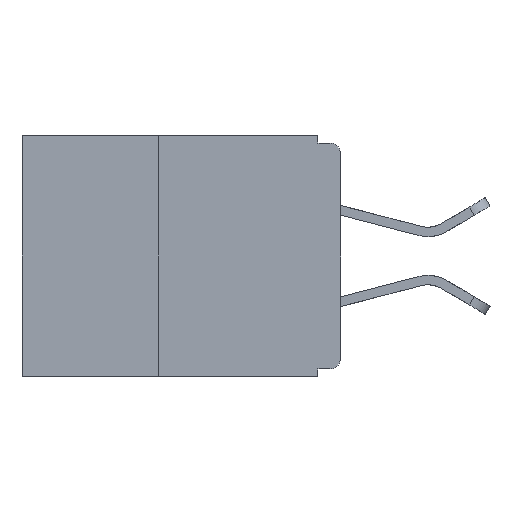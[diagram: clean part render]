
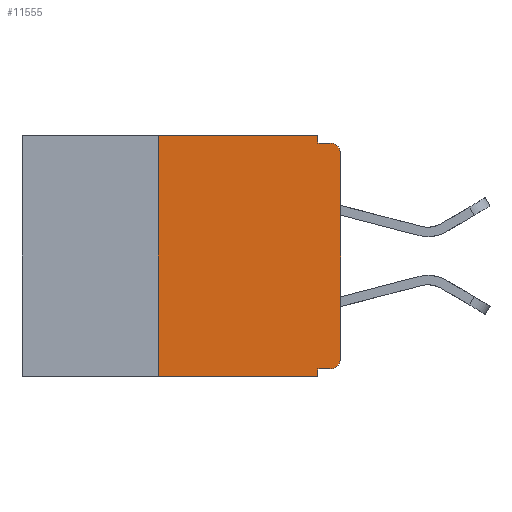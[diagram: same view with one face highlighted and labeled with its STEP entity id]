
A CAD part, left-side view. The second image highlights one B-rep face of the part: STEP entity #11555.
In plain terms, the highlighted planar face has unit normal (-1, 0, 0).
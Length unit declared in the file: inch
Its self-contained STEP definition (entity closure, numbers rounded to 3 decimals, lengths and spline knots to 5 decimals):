
#60 = LINE ( 'NONE', #8432, #3151 ) ;
#147 = ORIENTED_EDGE ( 'NONE', *, *, #15149, .F. ) ;
#393 = ORIENTED_EDGE ( 'NONE', *, *, #1273, .F. ) ;
#657 = VERTEX_POINT ( 'NONE', #5292 ) ;
#815 = LINE ( 'NONE', #12244, #10987 ) ;
#830 = LINE ( 'NONE', #1313, #14012 ) ;
#831 = EDGE_CURVE ( 'NONE', #12390, #9923, #12982, .T. ) ;
#835 = ORIENTED_EDGE ( 'NONE', *, *, #831, .F. ) ;
#950 = VERTEX_POINT ( 'NONE', #1779 ) ;
#1273 = EDGE_CURVE ( 'NONE', #950, #1953, #5854, .T. ) ;
#1313 = CARTESIAN_POINT ( 'NONE',  ( 0., 0., 0. ) ) ;
#1663 = DIRECTION ( 'NONE',  ( 0., 0., 1. ) ) ;
#1669 = CARTESIAN_POINT ( 'NONE',  ( 0., 0.25, -0.33 ) ) ;
#1736 = VERTEX_POINT ( 'NONE', #4764 ) ;
#1779 = CARTESIAN_POINT ( 'NONE',  ( 0., 0.25, -0.33 ) ) ;
#1802 = AXIS2_PLACEMENT_3D ( 'NONE', #13967, #6229, #15220 ) ;
#1953 = VERTEX_POINT ( 'NONE', #15444 ) ;
#2149 = AXIS2_PLACEMENT_3D ( 'NONE', #5535, #14590, #6918 ) ;
#2573 = ORIENTED_EDGE ( 'NONE', *, *, #5600, .F. ) ;
#2641 = VECTOR ( 'NONE', #1663, 39.37008 ) ;
#2836 = VECTOR ( 'NONE', #6023, 39.37008 ) ;
#2858 = VECTOR ( 'NONE', #7514, 39.37008 ) ;
#2935 = VERTEX_POINT ( 'NONE', #8820 ) ;
#3151 = VECTOR ( 'NONE', #12302, 39.37008 ) ;
#3494 = DIRECTION ( 'NONE',  ( 0., -1., 0. ) ) ;
#3678 = CARTESIAN_POINT ( 'NONE',  ( 0., 0.437, 0. ) ) ;
#3709 = FACE_OUTER_BOUND ( 'NONE', #16838, .T. ) ;
#4059 = ORIENTED_EDGE ( 'NONE', *, *, #11598, .F. ) ;
#4067 = EDGE_CURVE ( 'NONE', #2935, #12390, #14760, .T. ) ;
#4764 = CARTESIAN_POINT ( 'NONE',  ( 0., 0., -0.025 ) ) ;
#4772 = CARTESIAN_POINT ( 'NONE',  ( 0., 0., -0.32 ) ) ;
#4824 = EDGE_CURVE ( 'NONE', #950, #12009, #815, .T. ) ;
#5214 = CARTESIAN_POINT ( 'NONE',  ( 0., 0.437, 0. ) ) ;
#5292 = CARTESIAN_POINT ( 'NONE',  ( 0., 0., -0.305 ) ) ;
#5347 = VERTEX_POINT ( 'NONE', #6238 ) ;
#5535 = CARTESIAN_POINT ( 'NONE',  ( 0., 0.015, -0.025 ) ) ;
#5600 = EDGE_CURVE ( 'NONE', #1953, #2935, #9968, .T. ) ;
#5854 = LINE ( 'NONE', #1669, #2641 ) ;
#6023 = DIRECTION ( 'NONE',  ( 0., -1., 0. ) ) ;
#6229 = DIRECTION ( 'NONE',  ( -1., 0., 0. ) ) ;
#6238 = CARTESIAN_POINT ( 'NONE',  ( 0., 0.031, -0.32 ) ) ;
#6611 = DIRECTION ( 'NONE',  ( 0., 0., -1. ) ) ;
#6918 = DIRECTION ( 'NONE',  ( 0., 0., -1. ) ) ;
#7514 = DIRECTION ( 'NONE',  ( 0., 1., 0. ) ) ;
#8150 = CARTESIAN_POINT ( 'NONE',  ( 0., 0.015, -0.01 ) ) ;
#8239 = EDGE_CURVE ( 'NONE', #1736, #9923, #14835, .T. ) ;
#8432 = CARTESIAN_POINT ( 'NONE',  ( 0., 0.031, -0.33 ) ) ;
#8820 = CARTESIAN_POINT ( 'NONE',  ( 0., 0.031, 0. ) ) ;
#8836 = DIRECTION ( 'NONE',  ( 0., 0., -1. ) ) ;
#9342 = CARTESIAN_POINT ( 'NONE',  ( 0., 0.031, 0. ) ) ;
#9404 = DIRECTION ( 'NONE',  ( 0., 0., 1. ) ) ;
#9923 = VERTEX_POINT ( 'NONE', #8150 ) ;
#9968 = LINE ( 'NONE', #3678, #16335 ) ;
#10409 = CARTESIAN_POINT ( 'NONE',  ( 0., 0.031, -0.01 ) ) ;
#10707 = CARTESIAN_POINT ( 'NONE',  ( 0., 0.015, -0.32 ) ) ;
#10987 = VECTOR ( 'NONE', #11987, 39.37008 ) ;
#11026 = EDGE_CURVE ( 'NONE', #657, #1736, #830, .T. ) ;
#11207 = ORIENTED_EDGE ( 'NONE', *, *, #15332, .T. ) ;
#11287 = ORIENTED_EDGE ( 'NONE', *, *, #11026, .T. ) ;
#11555 = ADVANCED_FACE ( 'NONE', ( #3709 ), #13061, .F. ) ;
#11598 = EDGE_CURVE ( 'NONE', #16954, #5347, #13387, .T. ) ;
#11987 = DIRECTION ( 'NONE',  ( 0., -1., 0. ) ) ;
#12009 = VERTEX_POINT ( 'NONE', #12106 ) ;
#12106 = CARTESIAN_POINT ( 'NONE',  ( 0., 0.031, -0.33 ) ) ;
#12173 = CARTESIAN_POINT ( 'NONE',  ( 0., 0., -0.01 ) ) ;
#12244 = CARTESIAN_POINT ( 'NONE',  ( 0., 0.437, -0.33 ) ) ;
#12302 = DIRECTION ( 'NONE',  ( 0., 0., -1. ) ) ;
#12390 = VERTEX_POINT ( 'NONE', #10409 ) ;
#12634 = AXIS2_PLACEMENT_3D ( 'NONE', #5214, #14297, #6611 ) ;
#12713 = ORIENTED_EDGE ( 'NONE', *, *, #8239, .T. ) ;
#12982 = LINE ( 'NONE', #12173, #2836 ) ;
#13061 = PLANE ( 'NONE',  #12634 ) ;
#13387 = LINE ( 'NONE', #4772, #2858 ) ;
#13915 = ORIENTED_EDGE ( 'NONE', *, *, #4824, .T. ) ;
#13967 = CARTESIAN_POINT ( 'NONE',  ( 0., 0.015, -0.305 ) ) ;
#14012 = VECTOR ( 'NONE', #9404, 39.37008 ) ;
#14248 = CIRCLE ( 'NONE', #1802, 0.015 ) ;
#14297 = DIRECTION ( 'NONE',  ( 1., 0., 0. ) ) ;
#14376 = VECTOR ( 'NONE', #8836, 39.37008 ) ;
#14590 = DIRECTION ( 'NONE',  ( -1., 0., 0. ) ) ;
#14760 = LINE ( 'NONE', #9342, #14376 ) ;
#14835 = CIRCLE ( 'NONE', #2149, 0.015 ) ;
#15149 = EDGE_CURVE ( 'NONE', #5347, #12009, #60, .T. ) ;
#15220 = DIRECTION ( 'NONE',  ( 0., 0., -1. ) ) ;
#15332 = EDGE_CURVE ( 'NONE', #16954, #657, #14248, .T. ) ;
#15444 = CARTESIAN_POINT ( 'NONE',  ( 0., 0.25, 0. ) ) ;
#16335 = VECTOR ( 'NONE', #3494, 39.37008 ) ;
#16497 = ORIENTED_EDGE ( 'NONE', *, *, #4067, .F. ) ;
#16838 = EDGE_LOOP ( 'NONE', ( #11287, #12713, #835, #16497, #2573, #393, #13915, #147, #4059, #11207 ) ) ;
#16954 = VERTEX_POINT ( 'NONE', #10707 ) ;
